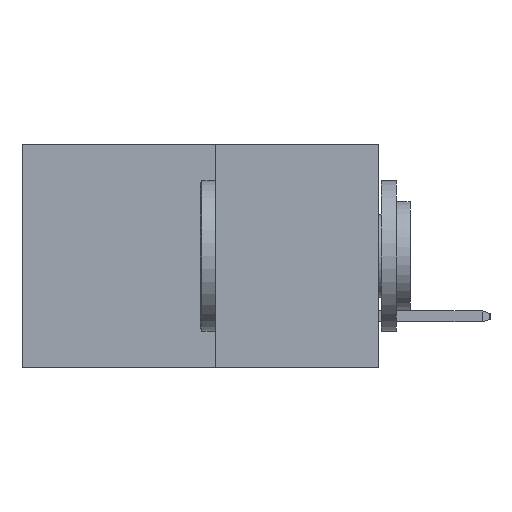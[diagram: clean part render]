
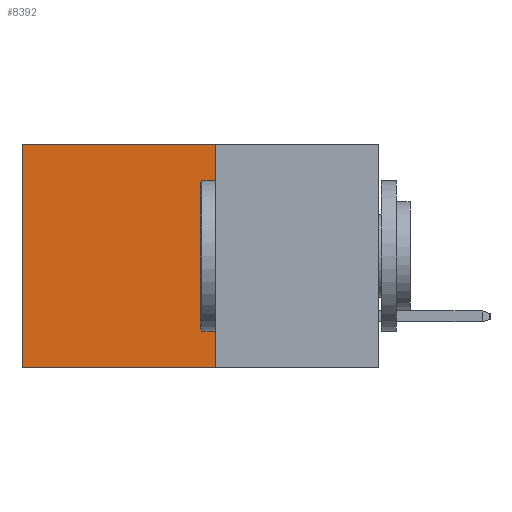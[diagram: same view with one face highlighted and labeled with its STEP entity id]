
A CAD part, left-side view. The second image highlights one B-rep face of the part: STEP entity #8392.
In plain terms, the highlighted planar face has unit normal (-1, 0, 0).
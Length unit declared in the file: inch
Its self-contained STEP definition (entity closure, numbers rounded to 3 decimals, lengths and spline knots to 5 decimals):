
#20 = CARTESIAN_POINT ( 'NONE',  ( 0.277, 0.27, 0. ) ) ;
#524 = EDGE_CURVE ( 'NONE', #642, #8644, #4190, .T. ) ;
#642 = VERTEX_POINT ( 'NONE', #20 ) ;
#1347 = DIRECTION ( 'NONE',  ( 0., 1., 0. ) ) ;
#1588 = DIRECTION ( 'NONE',  ( 0., 0., -1. ) ) ;
#1931 = VECTOR ( 'NONE', #6746, 39.37008 ) ;
#2667 = CARTESIAN_POINT ( 'NONE',  ( 0.277, 0.27, -0.37 ) ) ;
#2942 = ORIENTED_EDGE ( 'NONE', *, *, #6893, .F. ) ;
#3000 = EDGE_LOOP ( 'NONE', ( #5307, #5941, #2942, #3803 ) ) ;
#3359 = DIRECTION ( 'NONE',  ( 0., 0., -1. ) ) ;
#3439 = VERTEX_POINT ( 'NONE', #4603 ) ;
#3544 = VECTOR ( 'NONE', #1347, 39.37008 ) ;
#3731 = EDGE_CURVE ( 'NONE', #8644, #6902, #3781, .T. ) ;
#3781 = LINE ( 'NONE', #6992, #1931 ) ;
#3803 = ORIENTED_EDGE ( 'NONE', *, *, #524, .T. ) ;
#4190 = LINE ( 'NONE', #8419, #7603 ) ;
#4603 = CARTESIAN_POINT ( 'NONE',  ( 0.277, 0.27, -0.37 ) ) ;
#4661 = DIRECTION ( 'NONE',  ( 0., 1., 0. ) ) ;
#4689 = VECTOR ( 'NONE', #3359, 39.37008 ) ;
#4701 = AXIS2_PLACEMENT_3D ( 'NONE', #5696, #5729, #1588 ) ;
#5041 = PLANE ( 'NONE',  #4701 ) ;
#5307 = ORIENTED_EDGE ( 'NONE', *, *, #3731, .T. ) ;
#5585 = EDGE_CURVE ( 'NONE', #3439, #6902, #8520, .T. ) ;
#5696 = CARTESIAN_POINT ( 'NONE',  ( 0.277, 0.27, -0.37 ) ) ;
#5729 = DIRECTION ( 'NONE',  ( 1., 0., 0. ) ) ;
#5941 = ORIENTED_EDGE ( 'NONE', *, *, #5585, .F. ) ;
#6378 = FACE_OUTER_BOUND ( 'NONE', #3000, .T. ) ;
#6508 = LINE ( 'NONE', #2667, #4689 ) ;
#6746 = DIRECTION ( 'NONE',  ( 0., 0., -1. ) ) ;
#6893 = EDGE_CURVE ( 'NONE', #642, #3439, #6508, .T. ) ;
#6902 = VERTEX_POINT ( 'NONE', #7425 ) ;
#6992 = CARTESIAN_POINT ( 'NONE',  ( 0.277, 0.59, -0.37 ) ) ;
#7425 = CARTESIAN_POINT ( 'NONE',  ( 0.277, 0.59, -0.37 ) ) ;
#7603 = VECTOR ( 'NONE', #4661, 39.37008 ) ;
#7693 = CARTESIAN_POINT ( 'NONE',  ( 0.277, 0.27, -0.37 ) ) ;
#7949 = CARTESIAN_POINT ( 'NONE',  ( 0.277, 0.59, 0. ) ) ;
#8392 = ADVANCED_FACE ( 'NONE', ( #6378 ), #5041, .F. ) ;
#8419 = CARTESIAN_POINT ( 'NONE',  ( 0.277, 0.27, 0. ) ) ;
#8520 = LINE ( 'NONE', #7693, #3544 ) ;
#8644 = VERTEX_POINT ( 'NONE', #7949 ) ;
